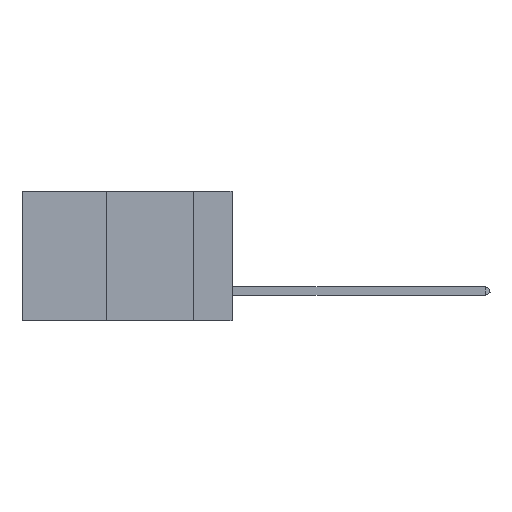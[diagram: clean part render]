
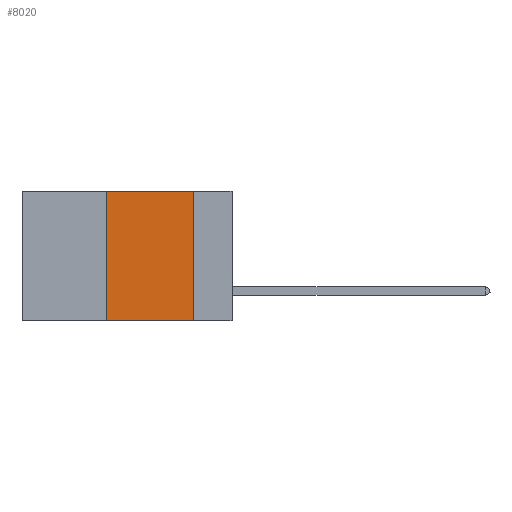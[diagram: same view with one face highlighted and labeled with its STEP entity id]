
A CAD part, left-side view. The second image highlights one B-rep face of the part: STEP entity #8020.
In plain terms, the highlighted planar face has unit normal (-1, 0, 0).
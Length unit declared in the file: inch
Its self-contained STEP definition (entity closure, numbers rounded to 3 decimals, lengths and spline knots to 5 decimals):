
#34 = VERTEX_POINT ( 'NONE', #9120 ) ;
#95 = VECTOR ( 'NONE', #10422, 39.37008 ) ;
#203 = FACE_OUTER_BOUND ( 'NONE', #2612, .T. ) ;
#240 = VERTEX_POINT ( 'NONE', #7727 ) ;
#324 = DIRECTION ( 'NONE',  ( 0., -1., 0. ) ) ;
#1153 = PLANE ( 'NONE',  #4059 ) ;
#1435 = VERTEX_POINT ( 'NONE', #2784 ) ;
#1610 = EDGE_CURVE ( 'NONE', #1435, #240, #2315, .T. ) ;
#2099 = LINE ( 'NONE', #2439, #7062 ) ;
#2315 = LINE ( 'NONE', #8875, #95 ) ;
#2439 = CARTESIAN_POINT ( 'NONE',  ( 0., 0.11, 0. ) ) ;
#2458 = EDGE_CURVE ( 'NONE', #240, #4689, #7114, .T. ) ;
#2612 = EDGE_LOOP ( 'NONE', ( #4713, #4665, #6312, #5743 ) ) ;
#2784 = CARTESIAN_POINT ( 'NONE',  ( 0., 0.36, -0.37 ) ) ;
#2822 = CARTESIAN_POINT ( 'NONE',  ( 0., 0.6, 0. ) ) ;
#4059 = AXIS2_PLACEMENT_3D ( 'NONE', #2822, #5339, #6169 ) ;
#4293 = LINE ( 'NONE', #9791, #8321 ) ;
#4626 = EDGE_CURVE ( 'NONE', #4689, #34, #2099, .T. ) ;
#4665 = ORIENTED_EDGE ( 'NONE', *, *, #2458, .F. ) ;
#4689 = VERTEX_POINT ( 'NONE', #5650 ) ;
#4713 = ORIENTED_EDGE ( 'NONE', *, *, #4626, .F. ) ;
#4841 = DIRECTION ( 'NONE',  ( 0., 0., -1. ) ) ;
#5323 = CARTESIAN_POINT ( 'NONE',  ( 0., 0.6, 0. ) ) ;
#5339 = DIRECTION ( 'NONE',  ( 1., 0., 0. ) ) ;
#5650 = CARTESIAN_POINT ( 'NONE',  ( 0., 0.11, 0. ) ) ;
#5743 = ORIENTED_EDGE ( 'NONE', *, *, #5876, .T. ) ;
#5876 = EDGE_CURVE ( 'NONE', #1435, #34, #4293, .T. ) ;
#6169 = DIRECTION ( 'NONE',  ( 0., 0., -1. ) ) ;
#6312 = ORIENTED_EDGE ( 'NONE', *, *, #1610, .F. ) ;
#7062 = VECTOR ( 'NONE', #4841, 39.37008 ) ;
#7114 = LINE ( 'NONE', #5323, #10450 ) ;
#7727 = CARTESIAN_POINT ( 'NONE',  ( 0., 0.36, 0. ) ) ;
#8020 = ADVANCED_FACE ( 'NONE', ( #203 ), #1153, .F. ) ;
#8321 = VECTOR ( 'NONE', #10621, 39.37008 ) ;
#8875 = CARTESIAN_POINT ( 'NONE',  ( 0., 0.36, 0. ) ) ;
#9120 = CARTESIAN_POINT ( 'NONE',  ( 0., 0.11, -0.37 ) ) ;
#9791 = CARTESIAN_POINT ( 'NONE',  ( 0., 0.6, -0.37 ) ) ;
#10422 = DIRECTION ( 'NONE',  ( 0., 0., 1. ) ) ;
#10450 = VECTOR ( 'NONE', #324, 39.37008 ) ;
#10621 = DIRECTION ( 'NONE',  ( 0., -1., 0. ) ) ;
